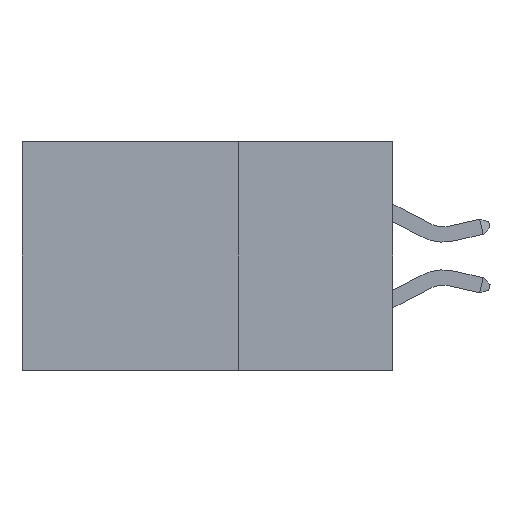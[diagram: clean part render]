
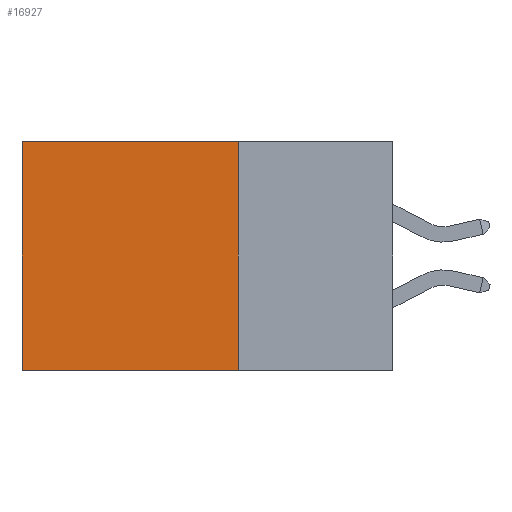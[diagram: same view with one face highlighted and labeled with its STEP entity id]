
A CAD part, left-side view. The second image highlights one B-rep face of the part: STEP entity #16927.
In plain terms, the highlighted planar face has unit normal (-1, 0, 0).
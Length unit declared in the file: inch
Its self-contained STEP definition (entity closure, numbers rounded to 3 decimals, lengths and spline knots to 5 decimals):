
#277 = DIRECTION ( 'NONE',  ( 0., 1., 0. ) ) ;
#712 = CARTESIAN_POINT ( 'NONE',  ( 0.2875, 0.25, -0.37 ) ) ;
#890 = VERTEX_POINT ( 'NONE', #1690 ) ;
#1690 = CARTESIAN_POINT ( 'NONE',  ( 0.2875, 0.25, -0.37 ) ) ;
#2278 = LINE ( 'NONE', #10555, #14135 ) ;
#2902 = VECTOR ( 'NONE', #277, 39.37008 ) ;
#3424 = VERTEX_POINT ( 'NONE', #7975 ) ;
#3719 = LINE ( 'NONE', #15468, #19692 ) ;
#3860 = DIRECTION ( 'NONE',  ( 1., 0., 0. ) ) ;
#4327 = AXIS2_PLACEMENT_3D ( 'NONE', #19235, #3860, #14728 ) ;
#4339 = CARTESIAN_POINT ( 'NONE',  ( 0.2875, 0.6, -0.37 ) ) ;
#6642 = EDGE_LOOP ( 'NONE', ( #15267, #8084, #12657, #8910 ) ) ;
#7490 = DIRECTION ( 'NONE',  ( 0., 0., -1. ) ) ;
#7975 = CARTESIAN_POINT ( 'NONE',  ( 0.2875, 0.6, 0. ) ) ;
#8063 = VECTOR ( 'NONE', #13141, 39.37008 ) ;
#8084 = ORIENTED_EDGE ( 'NONE', *, *, #9381, .F. ) ;
#8910 = ORIENTED_EDGE ( 'NONE', *, *, #9867, .T. ) ;
#9381 = EDGE_CURVE ( 'NONE', #890, #19267, #13120, .T. ) ;
#9867 = EDGE_CURVE ( 'NONE', #12316, #3424, #15250, .T. ) ;
#10555 = CARTESIAN_POINT ( 'NONE',  ( 0.2875, 0.6, 0. ) ) ;
#12316 = VERTEX_POINT ( 'NONE', #17699 ) ;
#12657 = ORIENTED_EDGE ( 'NONE', *, *, #13208, .F. ) ;
#13120 = LINE ( 'NONE', #712, #8063 ) ;
#13141 = DIRECTION ( 'NONE',  ( 0., 1., 0. ) ) ;
#13169 = PLANE ( 'NONE',  #4327 ) ;
#13208 = EDGE_CURVE ( 'NONE', #12316, #890, #3719, .T. ) ;
#13729 = EDGE_CURVE ( 'NONE', #3424, #19267, #2278, .T. ) ;
#14135 = VECTOR ( 'NONE', #7490, 39.37008 ) ;
#14728 = DIRECTION ( 'NONE',  ( 0., 0., -1. ) ) ;
#15250 = LINE ( 'NONE', #18852, #2902 ) ;
#15267 = ORIENTED_EDGE ( 'NONE', *, *, #13729, .T. ) ;
#15468 = CARTESIAN_POINT ( 'NONE',  ( 0.2875, 0.25, 0. ) ) ;
#16927 = ADVANCED_FACE ( 'NONE', ( #20042 ), #13169, .F. ) ;
#17006 = DIRECTION ( 'NONE',  ( 0., 0., -1. ) ) ;
#17699 = CARTESIAN_POINT ( 'NONE',  ( 0.2875, 0.25, 0. ) ) ;
#18852 = CARTESIAN_POINT ( 'NONE',  ( 0.2875, 0.25, 0. ) ) ;
#19235 = CARTESIAN_POINT ( 'NONE',  ( 0.2875, 0.25, 0. ) ) ;
#19267 = VERTEX_POINT ( 'NONE', #4339 ) ;
#19692 = VECTOR ( 'NONE', #17006, 39.37008 ) ;
#20042 = FACE_OUTER_BOUND ( 'NONE', #6642, .T. ) ;
